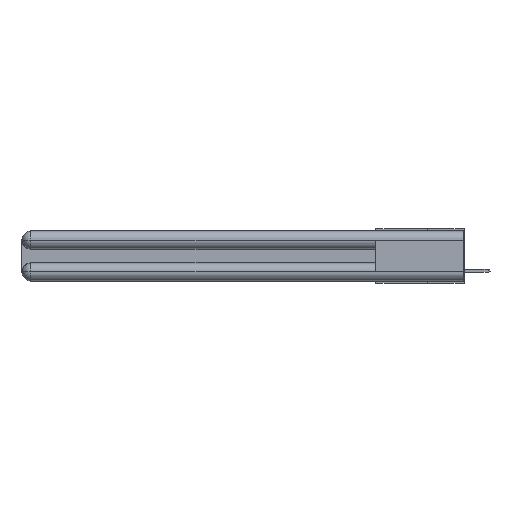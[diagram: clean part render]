
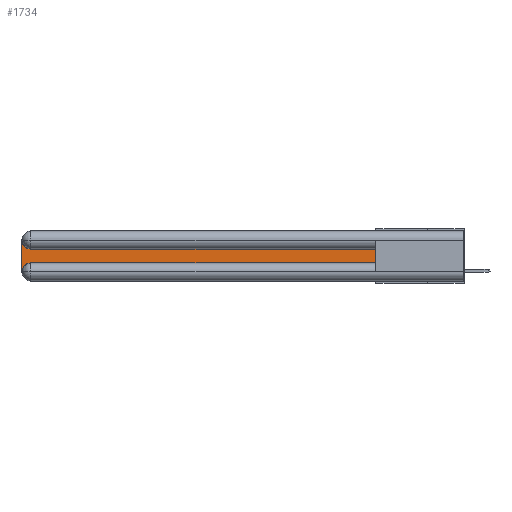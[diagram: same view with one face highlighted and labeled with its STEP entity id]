
A CAD part, left-side view. The second image highlights one B-rep face of the part: STEP entity #1734.
In plain terms, the highlighted planar face has unit normal (-1, 0, 0).
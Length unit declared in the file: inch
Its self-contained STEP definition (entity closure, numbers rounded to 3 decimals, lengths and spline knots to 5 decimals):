
#990 = DIRECTION ( 'NONE',  ( 1., 0., 0. ) ) ;
#1388 = VECTOR ( 'NONE', #13994, 39.37008 ) ;
#1734 = ADVANCED_FACE ( 'NONE', ( #6034 ), #31255, .F. ) ;
#1770 = AXIS2_PLACEMENT_3D ( 'NONE', #23700, #990, #3529 ) ;
#2416 = VECTOR ( 'NONE', #3699, 39.37008 ) ;
#2604 = CARTESIAN_POINT ( 'NONE',  ( 0.075, 3., -0.2175 ) ) ;
#3052 = DIRECTION ( 'NONE',  ( 0., -1., 0. ) ) ;
#3529 = DIRECTION ( 'NONE',  ( 0., 0., -1. ) ) ;
#3699 = DIRECTION ( 'NONE',  ( 0., 1., 0. ) ) ;
#4013 = ORIENTED_EDGE ( 'NONE', *, *, #6049, .T. ) ;
#5003 = CARTESIAN_POINT ( 'NONE',  ( 0.075, 2.94, -0.2775 ) ) ;
#6034 = FACE_OUTER_BOUND ( 'NONE', #26498, .T. ) ;
#6049 = EDGE_CURVE ( 'NONE', #12980, #26175, #10325, .T. ) ;
#7441 = CARTESIAN_POINT ( 'NONE',  ( 0.075, 3., -0.2775 ) ) ;
#7471 = DIRECTION ( 'NONE',  ( 0., 0., -1. ) ) ;
#7841 = VECTOR ( 'NONE', #12861, 39.37008 ) ;
#8048 = ORIENTED_EDGE ( 'NONE', *, *, #14593, .T. ) ;
#8075 = LINE ( 'NONE', #23933, #1388 ) ;
#9113 = ORIENTED_EDGE ( 'NONE', *, *, #10226, .T. ) ;
#9996 = LINE ( 'NONE', #26016, #17129 ) ;
#10226 = EDGE_CURVE ( 'NONE', #13422, #12984, #8075, .T. ) ;
#10325 = CIRCLE ( 'NONE', #23598, 0.06 ) ;
#10944 = CIRCLE ( 'NONE', #20982, 0.06 ) ;
#10959 = ORIENTED_EDGE ( 'NONE', *, *, #28480, .T. ) ;
#11671 = ORIENTED_EDGE ( 'NONE', *, *, #19831, .T. ) ;
#12155 = CARTESIAN_POINT ( 'NONE',  ( 0.075, 3., -0.0625 ) ) ;
#12861 = DIRECTION ( 'NONE',  ( 0., 0., -1. ) ) ;
#12980 = VERTEX_POINT ( 'NONE', #21979 ) ;
#12984 = VERTEX_POINT ( 'NONE', #21669 ) ;
#13422 = VERTEX_POINT ( 'NONE', #24073 ) ;
#13429 = EDGE_CURVE ( 'NONE', #12984, #12980, #16252, .T. ) ;
#13994 = DIRECTION ( 'NONE',  ( 0., 0., 1. ) ) ;
#14593 = EDGE_CURVE ( 'NONE', #26175, #19810, #21293, .T. ) ;
#16252 = LINE ( 'NONE', #17701, #2416 ) ;
#16400 = ORIENTED_EDGE ( 'NONE', *, *, #13429, .T. ) ;
#17129 = VECTOR ( 'NONE', #3052, 39.37008 ) ;
#17701 = CARTESIAN_POINT ( 'NONE',  ( 0.075, 0.6, -0.1225 ) ) ;
#17752 = DIRECTION ( 'NONE',  ( 1., 0., 0. ) ) ;
#18945 = VERTEX_POINT ( 'NONE', #24809 ) ;
#19701 = DIRECTION ( 'NONE',  ( 1., 0., 0. ) ) ;
#19810 = VERTEX_POINT ( 'NONE', #7441 ) ;
#19831 = EDGE_CURVE ( 'NONE', #19810, #18945, #10944, .T. ) ;
#20982 = AXIS2_PLACEMENT_3D ( 'NONE', #5003, #19701, #27744 ) ;
#21293 = LINE ( 'NONE', #2604, #7841 ) ;
#21669 = CARTESIAN_POINT ( 'NONE',  ( 0.075, 0.6, -0.1225 ) ) ;
#21979 = CARTESIAN_POINT ( 'NONE',  ( 0.075, 2.94, -0.1225 ) ) ;
#23598 = AXIS2_PLACEMENT_3D ( 'NONE', #24052, #17752, #7471 ) ;
#23700 = CARTESIAN_POINT ( 'NONE',  ( 0.075, 3., -0.1225 ) ) ;
#23933 = CARTESIAN_POINT ( 'NONE',  ( 0.075, 0.6, -0.2175 ) ) ;
#24052 = CARTESIAN_POINT ( 'NONE',  ( 0.075, 2.94, -0.0625 ) ) ;
#24073 = CARTESIAN_POINT ( 'NONE',  ( 0.075, 0.6, -0.2175 ) ) ;
#24809 = CARTESIAN_POINT ( 'NONE',  ( 0.075, 2.94, -0.2175 ) ) ;
#26016 = CARTESIAN_POINT ( 'NONE',  ( 0.075, 0.6, -0.2175 ) ) ;
#26175 = VERTEX_POINT ( 'NONE', #12155 ) ;
#26498 = EDGE_LOOP ( 'NONE', ( #16400, #4013, #8048, #11671, #10959, #9113 ) ) ;
#27744 = DIRECTION ( 'NONE',  ( 0., 0., -1. ) ) ;
#28480 = EDGE_CURVE ( 'NONE', #18945, #13422, #9996, .T. ) ;
#31255 = PLANE ( 'NONE',  #1770 ) ;
